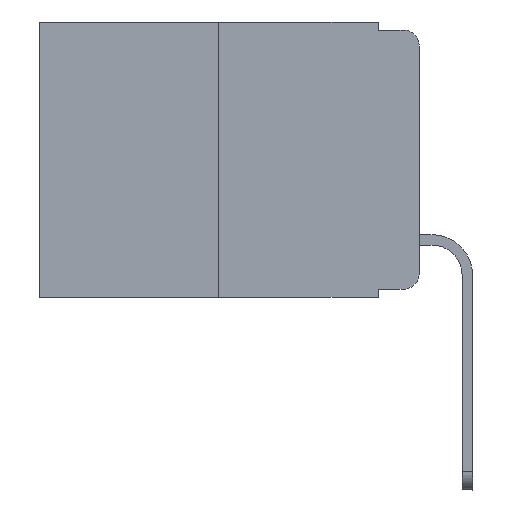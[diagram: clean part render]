
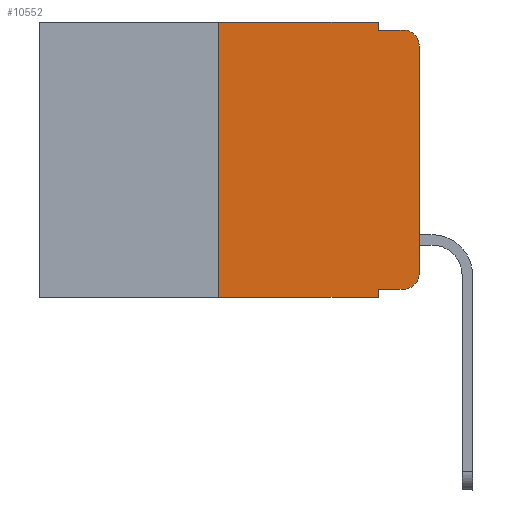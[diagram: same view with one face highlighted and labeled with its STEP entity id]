
A CAD part, left-side view. The second image highlights one B-rep face of the part: STEP entity #10552.
In plain terms, the highlighted planar face has unit normal (-1, 0, 0).
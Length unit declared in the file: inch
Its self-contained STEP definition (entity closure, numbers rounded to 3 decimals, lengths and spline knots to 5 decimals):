
#20 = LINE ( 'NONE', #13488, #2412 ) ;
#356 = ORIENTED_EDGE ( 'NONE', *, *, #11244, .F. ) ;
#583 = CARTESIAN_POINT ( 'NONE',  ( 0., 0.02, -0.333 ) ) ;
#632 = DIRECTION ( 'NONE',  ( 0., 0., -1. ) ) ;
#1199 = CARTESIAN_POINT ( 'NONE',  ( 0., 0.25, 0. ) ) ;
#1372 = CARTESIAN_POINT ( 'NONE',  ( 0., 0., 0. ) ) ;
#1583 = DIRECTION ( 'NONE',  ( -1., 0., 0. ) ) ;
#2104 = EDGE_CURVE ( 'NONE', #5564, #5320, #11471, .T. ) ;
#2367 = EDGE_LOOP ( 'NONE', ( #10001, #10978, #9218, #2569, #4630, #356, #12822, #10157, #12852, #9802 ) ) ;
#2412 = VECTOR ( 'NONE', #11221, 39.37008 ) ;
#2457 = LINE ( 'NONE', #2531, #12714 ) ;
#2531 = CARTESIAN_POINT ( 'NONE',  ( 0., 0.051, -0.01 ) ) ;
#2569 = ORIENTED_EDGE ( 'NONE', *, *, #6890, .F. ) ;
#2638 = LINE ( 'NONE', #8440, #14334 ) ;
#2711 = CARTESIAN_POINT ( 'NONE',  ( 0., 0.473, 0. ) ) ;
#2856 = CARTESIAN_POINT ( 'NONE',  ( 0., 0.051, 0. ) ) ;
#2909 = EDGE_CURVE ( 'NONE', #14560, #7181, #2457, .T. ) ;
#3159 = VECTOR ( 'NONE', #9628, 39.37008 ) ;
#3204 = DIRECTION ( 'NONE',  ( 0., 0., -1. ) ) ;
#3351 = VECTOR ( 'NONE', #8719, 39.37008 ) ;
#3821 = EDGE_CURVE ( 'NONE', #11913, #10674, #4935, .T. ) ;
#3898 = PLANE ( 'NONE',  #4748 ) ;
#4244 = LINE ( 'NONE', #8728, #11527 ) ;
#4306 = CARTESIAN_POINT ( 'NONE',  ( 0., 0.02, -0.03 ) ) ;
#4373 = VERTEX_POINT ( 'NONE', #7445 ) ;
#4480 = VECTOR ( 'NONE', #8246, 39.37008 ) ;
#4570 = LINE ( 'NONE', #1372, #13424 ) ;
#4630 = ORIENTED_EDGE ( 'NONE', *, *, #2104, .F. ) ;
#4688 = CARTESIAN_POINT ( 'NONE',  ( 0., 0.25, -0.343 ) ) ;
#4748 = AXIS2_PLACEMENT_3D ( 'NONE', #2711, #9624, #632 ) ;
#4935 = CIRCLE ( 'NONE', #13601, 0.02 ) ;
#5067 = DIRECTION ( 'NONE',  ( 0., 0., -1. ) ) ;
#5320 = VERTEX_POINT ( 'NONE', #9464 ) ;
#5564 = VERTEX_POINT ( 'NONE', #1199 ) ;
#5572 = VERTEX_POINT ( 'NONE', #6971 ) ;
#5675 = CIRCLE ( 'NONE', #8268, 0.02 ) ;
#5680 = CARTESIAN_POINT ( 'NONE',  ( 0., 0.473, 0. ) ) ;
#6160 = CARTESIAN_POINT ( 'NONE',  ( 0., 0.051, -0.01 ) ) ;
#6220 = EDGE_CURVE ( 'NONE', #5572, #7622, #9487, .T. ) ;
#6890 = EDGE_CURVE ( 'NONE', #5320, #14560, #9832, .T. ) ;
#6971 = CARTESIAN_POINT ( 'NONE',  ( 0., 0.051, -0.333 ) ) ;
#7181 = VERTEX_POINT ( 'NONE', #9971 ) ;
#7445 = CARTESIAN_POINT ( 'NONE',  ( 0., 0., -0.03 ) ) ;
#7622 = VERTEX_POINT ( 'NONE', #14030 ) ;
#7712 = DIRECTION ( 'NONE',  ( 0., -1., 0. ) ) ;
#8246 = DIRECTION ( 'NONE',  ( 0., -1., 0. ) ) ;
#8268 = AXIS2_PLACEMENT_3D ( 'NONE', #4306, #8793, #3204 ) ;
#8440 = CARTESIAN_POINT ( 'NONE',  ( 0., 0.051, -0.333 ) ) ;
#8719 = DIRECTION ( 'NONE',  ( 0., 0., -1. ) ) ;
#8728 = CARTESIAN_POINT ( 'NONE',  ( 0., 0.473, -0.343 ) ) ;
#8793 = DIRECTION ( 'NONE',  ( -1., 0., 0. ) ) ;
#9218 = ORIENTED_EDGE ( 'NONE', *, *, #2909, .F. ) ;
#9223 = DIRECTION ( 'NONE',  ( 0., -1., 0. ) ) ;
#9398 = CARTESIAN_POINT ( 'NONE',  ( 0., 0.02, -0.313 ) ) ;
#9436 = EDGE_CURVE ( 'NONE', #5572, #11913, #2638, .T. ) ;
#9464 = CARTESIAN_POINT ( 'NONE',  ( 0., 0.051, 0. ) ) ;
#9487 = LINE ( 'NONE', #2856, #3159 ) ;
#9575 = EDGE_CURVE ( 'NONE', #9603, #7622, #4244, .T. ) ;
#9603 = VERTEX_POINT ( 'NONE', #4688 ) ;
#9624 = DIRECTION ( 'NONE',  ( 1., 0., 0. ) ) ;
#9628 = DIRECTION ( 'NONE',  ( 0., 0., -1. ) ) ;
#9764 = CARTESIAN_POINT ( 'NONE',  ( 0., 0.051, 0. ) ) ;
#9802 = ORIENTED_EDGE ( 'NONE', *, *, #3821, .T. ) ;
#9832 = LINE ( 'NONE', #9764, #3351 ) ;
#9970 = EDGE_CURVE ( 'NONE', #4373, #7181, #5675, .T. ) ;
#9971 = CARTESIAN_POINT ( 'NONE',  ( 0., 0.02, -0.01 ) ) ;
#10001 = ORIENTED_EDGE ( 'NONE', *, *, #10486, .T. ) ;
#10157 = ORIENTED_EDGE ( 'NONE', *, *, #6220, .F. ) ;
#10360 = DIRECTION ( 'NONE',  ( 0., 0., 1. ) ) ;
#10486 = EDGE_CURVE ( 'NONE', #10674, #4373, #4570, .T. ) ;
#10552 = ADVANCED_FACE ( 'NONE', ( #12777 ), #3898, .F. ) ;
#10674 = VERTEX_POINT ( 'NONE', #13208 ) ;
#10978 = ORIENTED_EDGE ( 'NONE', *, *, #9970, .T. ) ;
#11221 = DIRECTION ( 'NONE',  ( 0., 0., 1. ) ) ;
#11244 = EDGE_CURVE ( 'NONE', #9603, #5564, #20, .T. ) ;
#11471 = LINE ( 'NONE', #5680, #4480 ) ;
#11527 = VECTOR ( 'NONE', #7712, 39.37008 ) ;
#11913 = VERTEX_POINT ( 'NONE', #583 ) ;
#12714 = VECTOR ( 'NONE', #9223, 39.37008 ) ;
#12777 = FACE_OUTER_BOUND ( 'NONE', #2367, .T. ) ;
#12822 = ORIENTED_EDGE ( 'NONE', *, *, #9575, .T. ) ;
#12840 = DIRECTION ( 'NONE',  ( 0., -1., 0. ) ) ;
#12852 = ORIENTED_EDGE ( 'NONE', *, *, #9436, .T. ) ;
#13208 = CARTESIAN_POINT ( 'NONE',  ( 0., 0., -0.313 ) ) ;
#13424 = VECTOR ( 'NONE', #10360, 39.37008 ) ;
#13488 = CARTESIAN_POINT ( 'NONE',  ( 0., 0.25, 0. ) ) ;
#13601 = AXIS2_PLACEMENT_3D ( 'NONE', #9398, #1583, #5067 ) ;
#14030 = CARTESIAN_POINT ( 'NONE',  ( 0., 0.051, -0.343 ) ) ;
#14334 = VECTOR ( 'NONE', #12840, 39.37008 ) ;
#14560 = VERTEX_POINT ( 'NONE', #6160 ) ;
